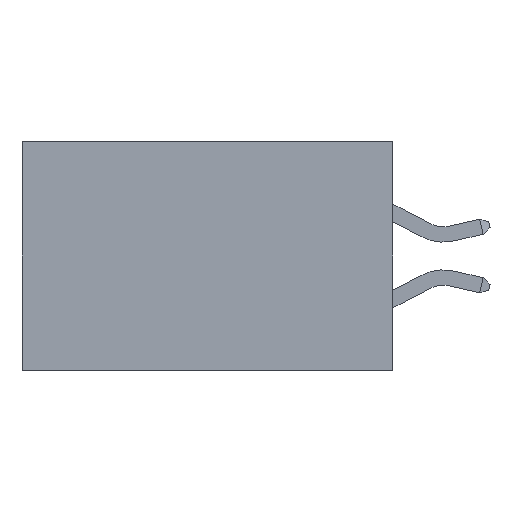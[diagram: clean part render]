
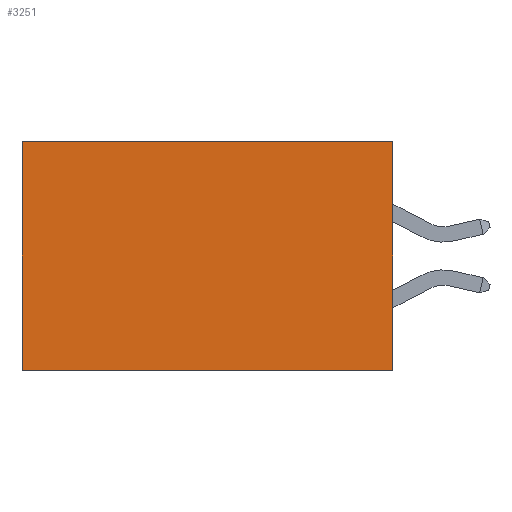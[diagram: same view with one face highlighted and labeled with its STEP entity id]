
A CAD part, left-side view. The second image highlights one B-rep face of the part: STEP entity #3251.
In plain terms, the highlighted planar face has unit normal (-1, 0, 0).
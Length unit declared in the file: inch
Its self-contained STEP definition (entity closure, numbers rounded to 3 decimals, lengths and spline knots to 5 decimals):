
#28 = CARTESIAN_POINT ( 'NONE',  ( 0.2875, 0., 0. ) ) ;
#543 = VERTEX_POINT ( 'NONE', #7111 ) ;
#916 = CARTESIAN_POINT ( 'NONE',  ( 0.2875, 0., -0.37 ) ) ;
#1045 = DIRECTION ( 'NONE',  ( 0., 1., 0. ) ) ;
#1396 = DIRECTION ( 'NONE',  ( 0., 0., -1. ) ) ;
#2153 = CARTESIAN_POINT ( 'NONE',  ( 0.2875, 0., 0. ) ) ;
#2242 = VERTEX_POINT ( 'NONE', #13073 ) ;
#3251 = ADVANCED_FACE ( 'NONE', ( #7116 ), #12819, .F. ) ;
#4054 = EDGE_CURVE ( 'NONE', #9877, #543, #18378, .T. ) ;
#4243 = DIRECTION ( 'NONE',  ( 1., 0., 0. ) ) ;
#4776 = EDGE_CURVE ( 'NONE', #9877, #2242, #18134, .T. ) ;
#5293 = EDGE_CURVE ( 'NONE', #2242, #12482, #16734, .T. ) ;
#5341 = VECTOR ( 'NONE', #10123, 39.37008 ) ;
#7076 = EDGE_LOOP ( 'NONE', ( #11939, #18286, #7661, #17066 ) ) ;
#7111 = CARTESIAN_POINT ( 'NONE',  ( 0.2875, 0.6, 0. ) ) ;
#7116 = FACE_OUTER_BOUND ( 'NONE', #7076, .T. ) ;
#7284 = CARTESIAN_POINT ( 'NONE',  ( 0.2875, 0., 0. ) ) ;
#7661 = ORIENTED_EDGE ( 'NONE', *, *, #4776, .F. ) ;
#8645 = VECTOR ( 'NONE', #12607, 39.37008 ) ;
#9092 = LINE ( 'NONE', #12367, #8645 ) ;
#9411 = EDGE_CURVE ( 'NONE', #543, #12482, #9092, .T. ) ;
#9877 = VERTEX_POINT ( 'NONE', #16188 ) ;
#10123 = DIRECTION ( 'NONE',  ( 0., 0., -1. ) ) ;
#10946 = VECTOR ( 'NONE', #13640, 39.37008 ) ;
#11232 = CARTESIAN_POINT ( 'NONE',  ( 0.2875, 0.6, -0.37 ) ) ;
#11939 = ORIENTED_EDGE ( 'NONE', *, *, #9411, .T. ) ;
#12367 = CARTESIAN_POINT ( 'NONE',  ( 0.2875, 0.6, 0. ) ) ;
#12482 = VERTEX_POINT ( 'NONE', #11232 ) ;
#12607 = DIRECTION ( 'NONE',  ( 0., 0., -1. ) ) ;
#12819 = PLANE ( 'NONE',  #14114 ) ;
#13073 = CARTESIAN_POINT ( 'NONE',  ( 0.2875, 0., -0.37 ) ) ;
#13640 = DIRECTION ( 'NONE',  ( 0., 1., 0. ) ) ;
#14114 = AXIS2_PLACEMENT_3D ( 'NONE', #28, #4243, #1396 ) ;
#16188 = CARTESIAN_POINT ( 'NONE',  ( 0.2875, 0., 0. ) ) ;
#16288 = VECTOR ( 'NONE', #1045, 39.37008 ) ;
#16734 = LINE ( 'NONE', #916, #16288 ) ;
#17066 = ORIENTED_EDGE ( 'NONE', *, *, #4054, .T. ) ;
#18134 = LINE ( 'NONE', #7284, #5341 ) ;
#18286 = ORIENTED_EDGE ( 'NONE', *, *, #5293, .F. ) ;
#18378 = LINE ( 'NONE', #2153, #10946 ) ;
